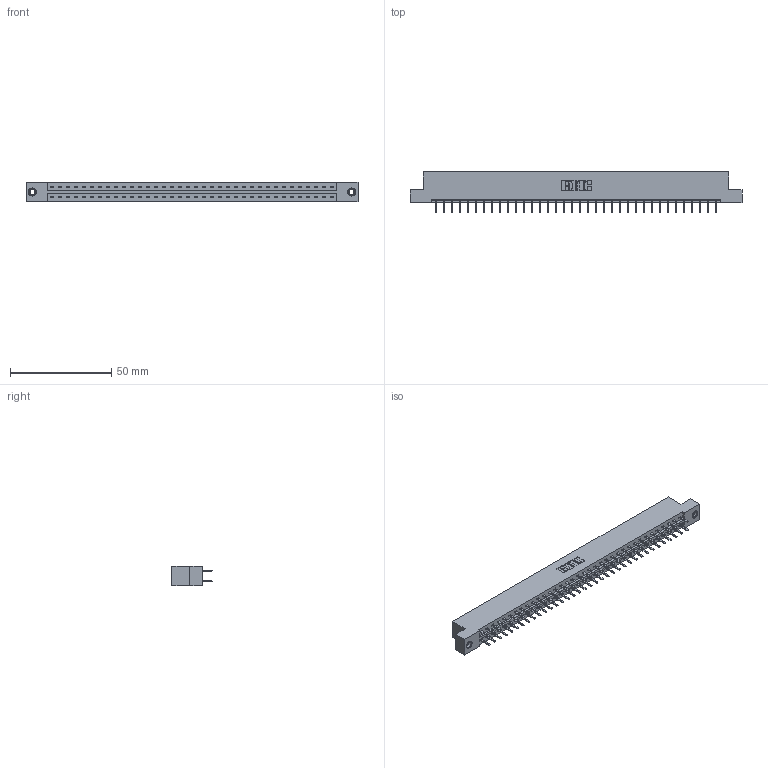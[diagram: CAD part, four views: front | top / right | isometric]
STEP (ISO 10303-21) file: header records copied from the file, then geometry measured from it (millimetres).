
FILE_DESCRIPTION (( 'STEP AP203' ), '1' );
FILE_NAME ('333-072-520-207.STEP', '2018-08-04T16:02:41', ( '' ), ( '' ), 'SwSTEP 2.0', 'SolidWorks 2016', '' );
FILE_SCHEMA (( 'CONFIG_CONTROL_DESIGN' ));
Length unit declared in the file: inch
Products named in the file (4): 333 Part_Flush - .156 Dia - TI; 345-292-001_345-293-120; 345-250-001_345-250-005-103; 333-072-520-207
Assembly tree (75 placements, depth 2):
  333-072-520-207
    333 Part_Flush - .156 Dia - TI
    345-292-001_345-293-120  x72
    345-250-001_345-250-005-103  x2
Bounding box: 164.19 x 20.02 x 9.4 mm (x, y, z)
Volume: 16661.1 mm3; surface area: 19583.4 mm2
Topology: 75 solids, 75 shells, 4206 faces, 12183 edges, 7922 vertices
Faces by surface type: plane 2838, cylinder 1352, cone 12, torus 4
Entity records: 25236 total; most frequent: CARTESIAN_POINT 4185, ORIENTED_EDGE 4102, DIRECTION 3605, EDGE_CURVE 2051, LINE 1899, VECTOR 1899, VERTEX_POINT 1360, AXIS2_PLACEMENT_3D 853
